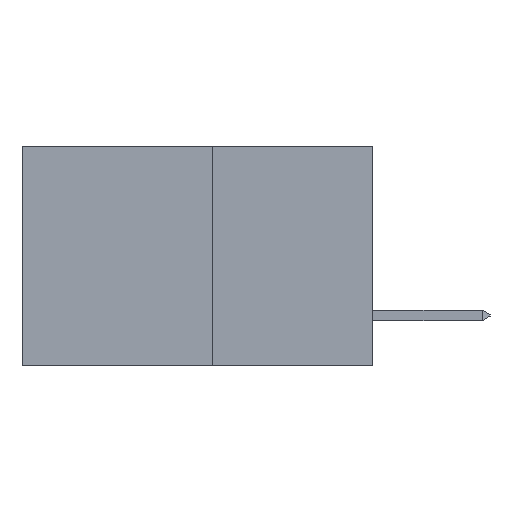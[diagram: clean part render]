
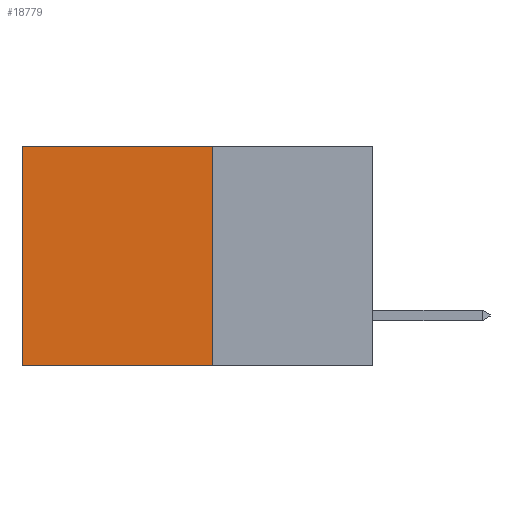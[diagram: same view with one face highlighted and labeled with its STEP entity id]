
A CAD part, left-side view. The second image highlights one B-rep face of the part: STEP entity #18779.
In plain terms, the highlighted planar face has unit normal (-1, 0, 0).
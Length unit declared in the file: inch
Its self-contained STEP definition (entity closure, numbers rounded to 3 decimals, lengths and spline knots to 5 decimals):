
#68 = DIRECTION ( 'NONE',  ( 0., 1., 0. ) ) ;
#567 = VECTOR ( 'NONE', #68, 39.37008 ) ;
#1416 = DIRECTION ( 'NONE',  ( 0., 1., 0. ) ) ;
#2044 = LINE ( 'NONE', #4965, #10463 ) ;
#2406 = LINE ( 'NONE', #3402, #20237 ) ;
#2437 = CARTESIAN_POINT ( 'NONE',  ( 0.277, 0.59, 0. ) ) ;
#3402 = CARTESIAN_POINT ( 'NONE',  ( 0.277, 0.59, -0.37 ) ) ;
#3643 = AXIS2_PLACEMENT_3D ( 'NONE', #5120, #10532, #22843 ) ;
#4121 = VERTEX_POINT ( 'NONE', #4544 ) ;
#4544 = CARTESIAN_POINT ( 'NONE',  ( 0.277, 0.27, 0. ) ) ;
#4965 = CARTESIAN_POINT ( 'NONE',  ( 0.277, 0.27, -0.37 ) ) ;
#5120 = CARTESIAN_POINT ( 'NONE',  ( 0.277, 0.27, -0.37 ) ) ;
#5311 = LINE ( 'NONE', #7185, #567 ) ;
#5851 = FACE_OUTER_BOUND ( 'NONE', #16865, .T. ) ;
#6764 = DIRECTION ( 'NONE',  ( 0., 0., -1. ) ) ;
#7185 = CARTESIAN_POINT ( 'NONE',  ( 0.277, 0.27, -0.37 ) ) ;
#7738 = EDGE_CURVE ( 'NONE', #14972, #11740, #2406, .T. ) ;
#8230 = CARTESIAN_POINT ( 'NONE',  ( 0.277, 0.59, -0.37 ) ) ;
#8372 = EDGE_CURVE ( 'NONE', #4121, #14972, #11616, .T. ) ;
#8719 = PLANE ( 'NONE',  #3643 ) ;
#9378 = ORIENTED_EDGE ( 'NONE', *, *, #8372, .T. ) ;
#10463 = VECTOR ( 'NONE', #6764, 39.37008 ) ;
#10532 = DIRECTION ( 'NONE',  ( 1., 0., 0. ) ) ;
#11199 = EDGE_CURVE ( 'NONE', #4121, #20242, #2044, .T. ) ;
#11616 = LINE ( 'NONE', #15703, #16324 ) ;
#11740 = VERTEX_POINT ( 'NONE', #8230 ) ;
#12681 = ORIENTED_EDGE ( 'NONE', *, *, #22585, .F. ) ;
#13248 = ORIENTED_EDGE ( 'NONE', *, *, #11199, .F. ) ;
#14123 = DIRECTION ( 'NONE',  ( 0., 0., -1. ) ) ;
#14622 = CARTESIAN_POINT ( 'NONE',  ( 0.277, 0.27, -0.37 ) ) ;
#14972 = VERTEX_POINT ( 'NONE', #2437 ) ;
#15703 = CARTESIAN_POINT ( 'NONE',  ( 0.277, 0.27, 0. ) ) ;
#16324 = VECTOR ( 'NONE', #1416, 39.37008 ) ;
#16865 = EDGE_LOOP ( 'NONE', ( #20882, #12681, #13248, #9378 ) ) ;
#18779 = ADVANCED_FACE ( 'NONE', ( #5851 ), #8719, .F. ) ;
#20237 = VECTOR ( 'NONE', #14123, 39.37008 ) ;
#20242 = VERTEX_POINT ( 'NONE', #14622 ) ;
#20882 = ORIENTED_EDGE ( 'NONE', *, *, #7738, .T. ) ;
#22585 = EDGE_CURVE ( 'NONE', #20242, #11740, #5311, .T. ) ;
#22843 = DIRECTION ( 'NONE',  ( 0., 0., -1. ) ) ;
